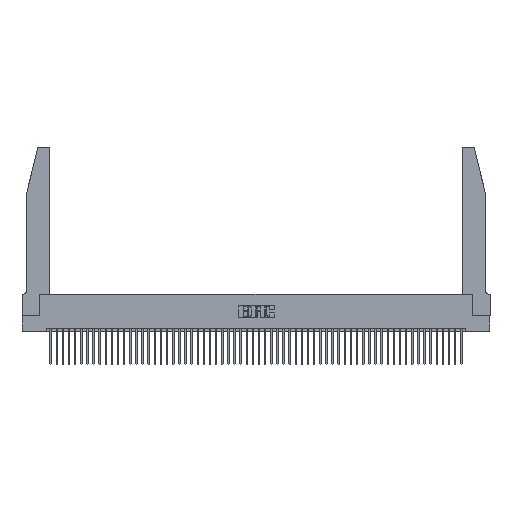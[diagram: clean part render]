
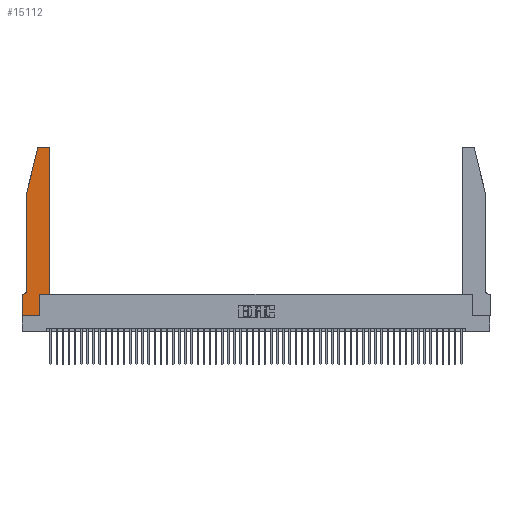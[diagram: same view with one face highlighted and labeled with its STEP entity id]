
A CAD part, top view. The second image highlights one B-rep face of the part: STEP entity #15112.
In plain terms, the highlighted planar face has unit normal (0, 0, 1).
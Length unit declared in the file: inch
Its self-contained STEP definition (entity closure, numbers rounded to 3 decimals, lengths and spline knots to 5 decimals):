
#144 = LINE ( 'NONE', #17055, #11545 ) ;
#166 = ORIENTED_EDGE ( 'NONE', *, *, #24051, .T. ) ;
#638 = VECTOR ( 'NONE', #18689, 39.37008 ) ;
#833 = EDGE_CURVE ( 'NONE', #11716, #29448, #144, .T. ) ;
#1683 = CARTESIAN_POINT ( 'NONE',  ( 0., 0., 0.37 ) ) ;
#1848 = LINE ( 'NONE', #33401, #24508 ) ;
#3117 = VERTEX_POINT ( 'NONE', #43627 ) ;
#3169 = EDGE_CURVE ( 'NONE', #3117, #11716, #23339, .T. ) ;
#4155 = DIRECTION ( 'NONE',  ( 1., 0., 0. ) ) ;
#4197 = ORIENTED_EDGE ( 'NONE', *, *, #17331, .T. ) ;
#5237 = DIRECTION ( 'NONE',  ( 0., -1., 0. ) ) ;
#5594 = DIRECTION ( 'NONE',  ( 0., 0., 1. ) ) ;
#7054 = ORIENTED_EDGE ( 'NONE', *, *, #18949, .T. ) ;
#7381 = PLANE ( 'NONE',  #43937 ) ;
#7627 = DIRECTION ( 'NONE',  ( 1., 0., 0. ) ) ;
#8001 = DIRECTION ( 'NONE',  ( -1., 0., 0. ) ) ;
#8794 = ORIENTED_EDGE ( 'NONE', *, *, #12982, .T. ) ;
#9708 = VERTEX_POINT ( 'NONE', #44699 ) ;
#10823 = CARTESIAN_POINT ( 'NONE',  ( 0.2865, 0.35, 0.37 ) ) ;
#11436 = EDGE_CURVE ( 'NONE', #33317, #27199, #47667, .T. ) ;
#11545 = VECTOR ( 'NONE', #4155, 39.37008 ) ;
#11565 = ORIENTED_EDGE ( 'NONE', *, *, #45291, .T. ) ;
#11693 = DIRECTION ( 'NONE',  ( 0., 0., 1. ) ) ;
#11716 = VERTEX_POINT ( 'NONE', #15687 ) ;
#11948 = CARTESIAN_POINT ( 'NONE',  ( 0.0755, 2., 0.37 ) ) ;
#12216 = LINE ( 'NONE', #11948, #54276 ) ;
#12472 = VECTOR ( 'NONE', #32095, 39.37008 ) ;
#12982 = EDGE_CURVE ( 'NONE', #9708, #33317, #44560, .T. ) ;
#13604 = ORIENTED_EDGE ( 'NONE', *, *, #833, .T. ) ;
#14524 = EDGE_CURVE ( 'NONE', #46401, #9708, #16838, .T. ) ;
#15112 = ADVANCED_FACE ( 'NONE', ( #32570 ), #7381, .T. ) ;
#15650 = VERTEX_POINT ( 'NONE', #52259 ) ;
#15687 = CARTESIAN_POINT ( 'NONE',  ( 0., 0., 0.37 ) ) ;
#16133 = CIRCLE ( 'NONE', #40608, 0.07 ) ;
#16204 = ORIENTED_EDGE ( 'NONE', *, *, #11436, .T. ) ;
#16838 = LINE ( 'NONE', #28812, #26701 ) ;
#17055 = CARTESIAN_POINT ( 'NONE',  ( 0., 0., 0.37 ) ) ;
#17331 = EDGE_CURVE ( 'NONE', #29448, #46401, #23786, .T. ) ;
#18689 = DIRECTION ( 'NONE',  ( 0., -1., 0. ) ) ;
#18949 = EDGE_CURVE ( 'NONE', #21925, #15650, #43196, .T. ) ;
#19348 = EDGE_CURVE ( 'NONE', #30666, #21925, #12216, .T. ) ;
#20526 = VECTOR ( 'NONE', #41504, 39.37008 ) ;
#20585 = CARTESIAN_POINT ( 'NONE',  ( 0.0755, 0.35, 0.37 ) ) ;
#20700 = DIRECTION ( 'NONE',  ( -0.239, -0.971, 0. ) ) ;
#20914 = VECTOR ( 'NONE', #5237, 39.37008 ) ;
#21045 = CARTESIAN_POINT ( 'NONE',  ( 0.0755, 2., 0.37 ) ) ;
#21840 = LINE ( 'NONE', #20585, #20526 ) ;
#21925 = VERTEX_POINT ( 'NONE', #21045 ) ;
#22195 = CARTESIAN_POINT ( 'NONE',  ( 0.0055, 0.42, 0.37 ) ) ;
#22680 = CARTESIAN_POINT ( 'NONE',  ( 0.284, 2.72, 0.37 ) ) ;
#23339 = LINE ( 'NONE', #1683, #638 ) ;
#23491 = AXIS2_PLACEMENT_3D ( 'NONE', #31024, #5594, #35258 ) ;
#23786 = LINE ( 'NONE', #10823, #12472 ) ;
#23849 = ORIENTED_EDGE ( 'NONE', *, *, #36914, .T. ) ;
#24051 = EDGE_CURVE ( 'NONE', #50969, #30666, #30954, .T. ) ;
#24382 = ORIENTED_EDGE ( 'NONE', *, *, #19348, .T. ) ;
#24508 = VECTOR ( 'NONE', #8001, 39.37008 ) ;
#26350 = EDGE_CURVE ( 'NONE', #27199, #50969, #1848, .T. ) ;
#26394 = DIRECTION ( 'NONE',  ( -1., 0., 0. ) ) ;
#26701 = VECTOR ( 'NONE', #7627, 39.37008 ) ;
#26882 = DIRECTION ( 'NONE',  ( 1., 0., 0. ) ) ;
#27199 = VERTEX_POINT ( 'NONE', #43337 ) ;
#28812 = CARTESIAN_POINT ( 'NONE',  ( 0.4505, 0.35, 0.37 ) ) ;
#29182 = CARTESIAN_POINT ( 'NONE',  ( 0.2865, 0.35, 0.37 ) ) ;
#29448 = VERTEX_POINT ( 'NONE', #43256 ) ;
#29752 = VERTEX_POINT ( 'NONE', #36694 ) ;
#30666 = VERTEX_POINT ( 'NONE', #32139 ) ;
#30954 = CIRCLE ( 'NONE', #52261, 0.03 ) ;
#31024 = CARTESIAN_POINT ( 'NONE',  ( 0.4205, 2.72, 0.37 ) ) ;
#32095 = DIRECTION ( 'NONE',  ( 0., 1., 0. ) ) ;
#32139 = CARTESIAN_POINT ( 'NONE',  ( 0.25487, 2.72718, 0.37 ) ) ;
#32265 = CARTESIAN_POINT ( 'NONE',  ( 0.4505, 2.72, 0.37 ) ) ;
#32570 = FACE_OUTER_BOUND ( 'NONE', #41484, .T. ) ;
#32700 = ORIENTED_EDGE ( 'NONE', *, *, #14524, .T. ) ;
#33317 = VERTEX_POINT ( 'NONE', #32265 ) ;
#33401 = CARTESIAN_POINT ( 'NONE',  ( 0.2605, 2.75, 0.37 ) ) ;
#33478 = VECTOR ( 'NONE', #48114, 39.37008 ) ;
#34880 = CARTESIAN_POINT ( 'NONE',  ( 0.0755, 2., 0.37 ) ) ;
#35258 = DIRECTION ( 'NONE',  ( 1., 0., 0. ) ) ;
#36088 = ORIENTED_EDGE ( 'NONE', *, *, #26350, .T. ) ;
#36694 = CARTESIAN_POINT ( 'NONE',  ( 0.0055, 0.35, 0.37 ) ) ;
#36914 = EDGE_CURVE ( 'NONE', #29752, #3117, #21840, .T. ) ;
#40608 = AXIS2_PLACEMENT_3D ( 'NONE', #22195, #51469, #26394 ) ;
#41192 = DIRECTION ( 'NONE',  ( 1., 0., 0. ) ) ;
#41484 = EDGE_LOOP ( 'NONE', ( #36088, #166, #24382, #7054, #11565, #23849, #47781, #13604, #4197, #32700, #8794, #16204 ) ) ;
#41504 = DIRECTION ( 'NONE',  ( -1., 0., 0. ) ) ;
#43196 = LINE ( 'NONE', #34880, #20914 ) ;
#43256 = CARTESIAN_POINT ( 'NONE',  ( 0.2865, 0., 0.37 ) ) ;
#43337 = CARTESIAN_POINT ( 'NONE',  ( 0.4205, 2.75, 0.37 ) ) ;
#43627 = CARTESIAN_POINT ( 'NONE',  ( 0., 0.35, 0.37 ) ) ;
#43923 = CARTESIAN_POINT ( 'NONE',  ( 0.4505, 0.35, 0.37 ) ) ;
#43937 = AXIS2_PLACEMENT_3D ( 'NONE', #49400, #11693, #41192 ) ;
#44560 = LINE ( 'NONE', #43923, #33478 ) ;
#44699 = CARTESIAN_POINT ( 'NONE',  ( 0.4505, 0.35, 0.37 ) ) ;
#45291 = EDGE_CURVE ( 'NONE', #15650, #29752, #16133, .T. ) ;
#46401 = VERTEX_POINT ( 'NONE', #29182 ) ;
#47667 = CIRCLE ( 'NONE', #23491, 0.03 ) ;
#47781 = ORIENTED_EDGE ( 'NONE', *, *, #3169, .T. ) ;
#48114 = DIRECTION ( 'NONE',  ( 0., 1., 0. ) ) ;
#49400 = CARTESIAN_POINT ( 'NONE',  ( 0., 0.35, 0.37 ) ) ;
#50969 = VERTEX_POINT ( 'NONE', #51333 ) ;
#51333 = CARTESIAN_POINT ( 'NONE',  ( 0.284, 2.75, 0.37 ) ) ;
#51469 = DIRECTION ( 'NONE',  ( 0., 0., -1. ) ) ;
#51940 = DIRECTION ( 'NONE',  ( 0., 0., 1. ) ) ;
#52259 = CARTESIAN_POINT ( 'NONE',  ( 0.0755, 0.42, 0.37 ) ) ;
#52261 = AXIS2_PLACEMENT_3D ( 'NONE', #22680, #51940, #26882 ) ;
#54276 = VECTOR ( 'NONE', #20700, 39.37008 ) ;
